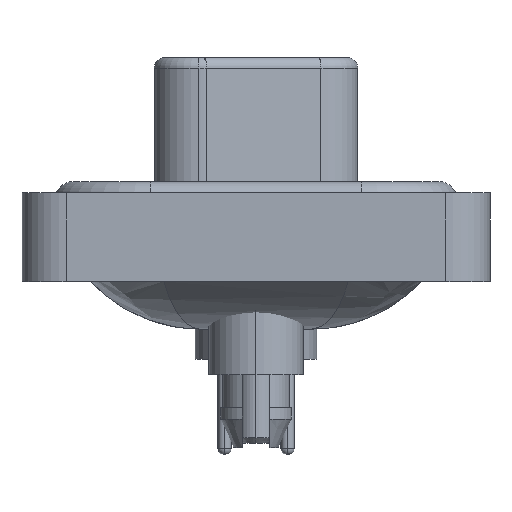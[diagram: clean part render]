
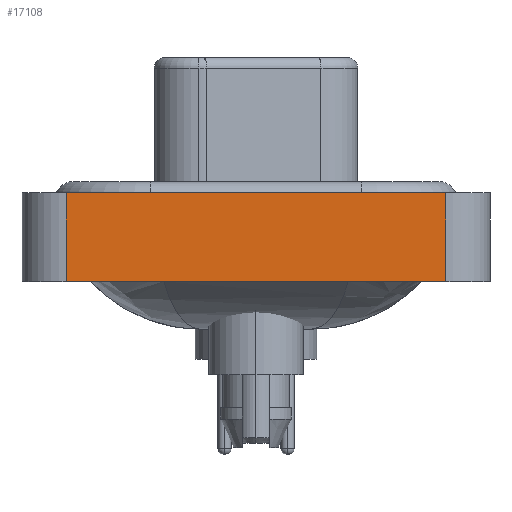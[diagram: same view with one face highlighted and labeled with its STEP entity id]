
A CAD part, left-side view. The second image highlights one B-rep face of the part: STEP entity #17108.
In plain terms, the highlighted planar face has unit normal (-1, 0, 0).
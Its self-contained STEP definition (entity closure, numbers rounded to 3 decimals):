
#554 = DIRECTION ( 'NONE',  ( -1., 0., 0. ) ) ;
#983 = VERTEX_POINT ( 'NONE', #8543 ) ;
#1151 = AXIS2_PLACEMENT_3D ( 'NONE', #2207, #554, #10331 ) ;
#1459 = CARTESIAN_POINT ( 'NONE',  ( -7.35, -8.55, 0.4 ) ) ;
#2009 = EDGE_LOOP ( 'NONE', ( #7785, #11516, #6871, #6795 ) ) ;
#2207 = CARTESIAN_POINT ( 'NONE',  ( -7.35, -8.55, -3.6 ) ) ;
#2245 = EDGE_CURVE ( 'NONE', #17676, #3717, #16540, .T. ) ;
#2718 = EDGE_CURVE ( 'NONE', #18312, #983, #11677, .T. ) ;
#3717 = VERTEX_POINT ( 'NONE', #9900 ) ;
#4046 = CARTESIAN_POINT ( 'NONE',  ( -7.35, 8.55, -3.6 ) ) ;
#5051 = VECTOR ( 'NONE', #10256, 1000. ) ;
#5100 = CARTESIAN_POINT ( 'NONE',  ( -7.35, -8.55, -3.6 ) ) ;
#6676 = DIRECTION ( 'NONE',  ( 0., 0., 1. ) ) ;
#6795 = ORIENTED_EDGE ( 'NONE', *, *, #2245, .T. ) ;
#6871 = ORIENTED_EDGE ( 'NONE', *, *, #9439, .F. ) ;
#7785 = ORIENTED_EDGE ( 'NONE', *, *, #18797, .T. ) ;
#7824 = LINE ( 'NONE', #21017, #8187 ) ;
#8187 = VECTOR ( 'NONE', #6676, 1000. ) ;
#8543 = CARTESIAN_POINT ( 'NONE',  ( -7.35, -8.55, 0.4 ) ) ;
#9439 = EDGE_CURVE ( 'NONE', #17676, #18312, #21232, .T. ) ;
#9900 = CARTESIAN_POINT ( 'NONE',  ( -7.35, -8.55, -3.6 ) ) ;
#10256 = DIRECTION ( 'NONE',  ( 0., -1., 0. ) ) ;
#10331 = DIRECTION ( 'NONE',  ( 0., 0., 1. ) ) ;
#11224 = CARTESIAN_POINT ( 'NONE',  ( -7.35, 8.55, -3.6 ) ) ;
#11481 = CARTESIAN_POINT ( 'NONE',  ( -7.35, 8.55, 0.4 ) ) ;
#11516 = ORIENTED_EDGE ( 'NONE', *, *, #2718, .F. ) ;
#11677 = LINE ( 'NONE', #1459, #21226 ) ;
#13614 = FACE_OUTER_BOUND ( 'NONE', #2009, .T. ) ;
#16234 = VECTOR ( 'NONE', #17918, 1000. ) ;
#16540 = LINE ( 'NONE', #5100, #5051 ) ;
#16622 = DIRECTION ( 'NONE',  ( 0., -1., 0. ) ) ;
#17108 = ADVANCED_FACE ( 'NONE', ( #13614 ), #20436, .T. ) ;
#17676 = VERTEX_POINT ( 'NONE', #4046 ) ;
#17918 = DIRECTION ( 'NONE',  ( 0., 0., 1. ) ) ;
#18312 = VERTEX_POINT ( 'NONE', #11481 ) ;
#18797 = EDGE_CURVE ( 'NONE', #3717, #983, #7824, .T. ) ;
#20436 = PLANE ( 'NONE',  #1151 ) ;
#21017 = CARTESIAN_POINT ( 'NONE',  ( -7.35, -8.55, -3.6 ) ) ;
#21226 = VECTOR ( 'NONE', #16622, 1000. ) ;
#21232 = LINE ( 'NONE', #11224, #16234 ) ;
